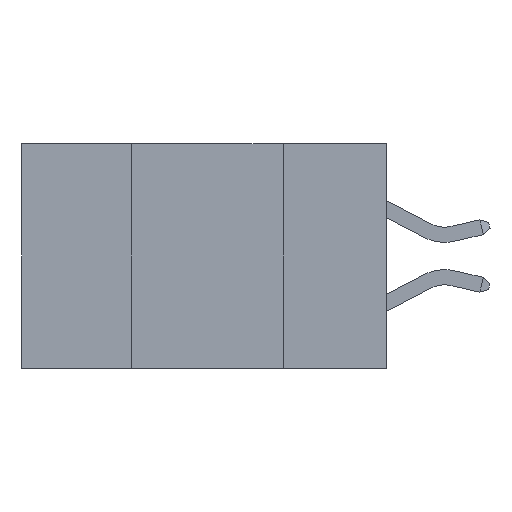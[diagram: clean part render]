
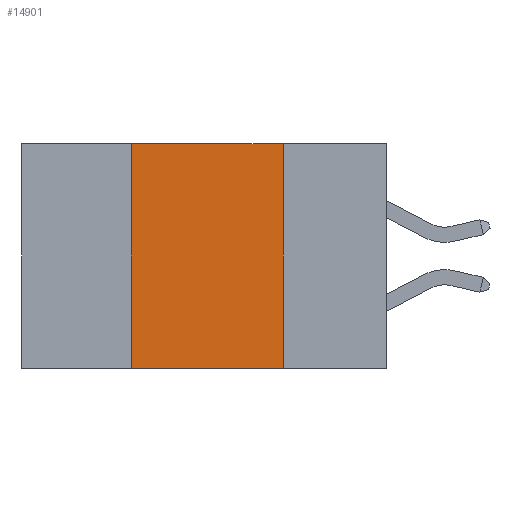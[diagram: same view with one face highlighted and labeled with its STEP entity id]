
A CAD part, left-side view. The second image highlights one B-rep face of the part: STEP entity #14901.
In plain terms, the highlighted planar face has unit normal (-1, 0, 0).
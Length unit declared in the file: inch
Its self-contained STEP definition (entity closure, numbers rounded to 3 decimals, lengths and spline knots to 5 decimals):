
#323 = CARTESIAN_POINT ( 'NONE',  ( 0., 0.42, -0.37 ) ) ;
#1484 = EDGE_CURVE ( 'NONE', #13561, #5809, #17837, .T. ) ;
#3009 = CARTESIAN_POINT ( 'NONE',  ( 0., 0.6, 0. ) ) ;
#4840 = ORIENTED_EDGE ( 'NONE', *, *, #19696, .T. ) ;
#4916 = CARTESIAN_POINT ( 'NONE',  ( 0., 0.17, 0. ) ) ;
#5809 = VERTEX_POINT ( 'NONE', #4916 ) ;
#6156 = CARTESIAN_POINT ( 'NONE',  ( 0., 0.17, -0.37 ) ) ;
#6170 = VERTEX_POINT ( 'NONE', #6156 ) ;
#6248 = PLANE ( 'NONE',  #16130 ) ;
#8586 = CARTESIAN_POINT ( 'NONE',  ( 0., 0.42, 0. ) ) ;
#8680 = DIRECTION ( 'NONE',  ( 0., 0., -1. ) ) ;
#9407 = DIRECTION ( 'NONE',  ( 0., -1., 0. ) ) ;
#9922 = CARTESIAN_POINT ( 'NONE',  ( 0., 0.42, 0. ) ) ;
#11078 = CARTESIAN_POINT ( 'NONE',  ( 0., 0.17, 0. ) ) ;
#11646 = EDGE_LOOP ( 'NONE', ( #24231, #27568, #29464, #4840 ) ) ;
#12561 = VECTOR ( 'NONE', #29380, 39.37008 ) ;
#13561 = VERTEX_POINT ( 'NONE', #8586 ) ;
#14849 = LINE ( 'NONE', #9922, #12561 ) ;
#14901 = ADVANCED_FACE ( 'NONE', ( #26745 ), #6248, .F. ) ;
#15234 = DIRECTION ( 'NONE',  ( 0., -1., 0. ) ) ;
#16130 = AXIS2_PLACEMENT_3D ( 'NONE', #30499, #23288, #8680 ) ;
#17837 = LINE ( 'NONE', #3009, #24365 ) ;
#18472 = VECTOR ( 'NONE', #15234, 39.37008 ) ;
#19696 = EDGE_CURVE ( 'NONE', #27208, #6170, #24978, .T. ) ;
#20853 = LINE ( 'NONE', #11078, #27329 ) ;
#23288 = DIRECTION ( 'NONE',  ( 1., 0., 0. ) ) ;
#24231 = ORIENTED_EDGE ( 'NONE', *, *, #30126, .F. ) ;
#24365 = VECTOR ( 'NONE', #9407, 39.37008 ) ;
#24404 = EDGE_CURVE ( 'NONE', #27208, #13561, #14849, .T. ) ;
#24978 = LINE ( 'NONE', #24984, #18472 ) ;
#24984 = CARTESIAN_POINT ( 'NONE',  ( 0., 0.6, -0.37 ) ) ;
#26745 = FACE_OUTER_BOUND ( 'NONE', #11646, .T. ) ;
#27208 = VERTEX_POINT ( 'NONE', #323 ) ;
#27329 = VECTOR ( 'NONE', #28134, 39.37008 ) ;
#27568 = ORIENTED_EDGE ( 'NONE', *, *, #1484, .F. ) ;
#28134 = DIRECTION ( 'NONE',  ( 0., 0., -1. ) ) ;
#29380 = DIRECTION ( 'NONE',  ( 0., 0., 1. ) ) ;
#29464 = ORIENTED_EDGE ( 'NONE', *, *, #24404, .F. ) ;
#30126 = EDGE_CURVE ( 'NONE', #5809, #6170, #20853, .T. ) ;
#30499 = CARTESIAN_POINT ( 'NONE',  ( 0., 0.6, 0. ) ) ;
